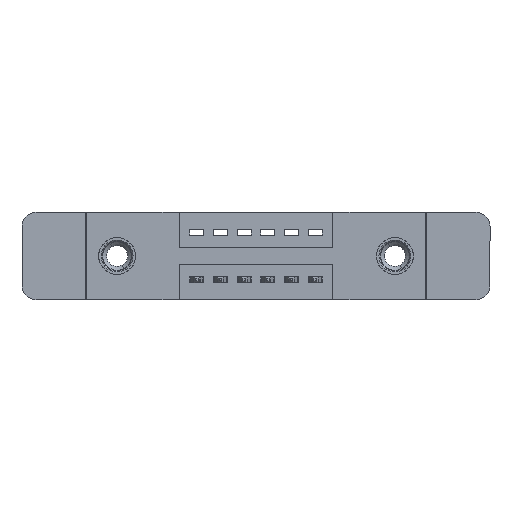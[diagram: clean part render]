
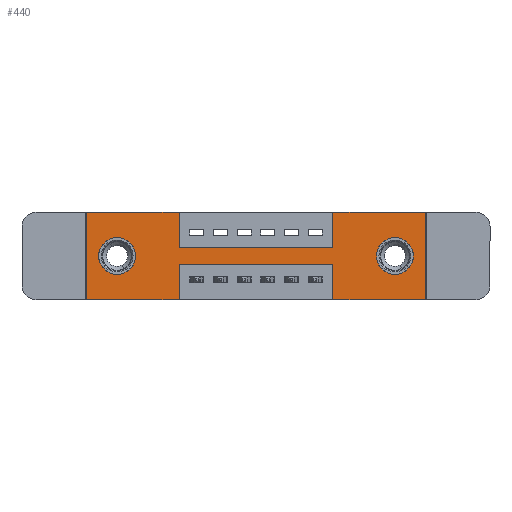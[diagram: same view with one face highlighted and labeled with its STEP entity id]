
A CAD part, front view. The second image highlights one B-rep face of the part: STEP entity #440.
In plain terms, the highlighted planar face has unit normal (0, -1, 0).
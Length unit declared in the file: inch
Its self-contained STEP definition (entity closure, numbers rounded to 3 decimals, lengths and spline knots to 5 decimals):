
#21 = DIRECTION ( 'NONE',  ( 0., 1., 0. ) ) ;
#76 = DIRECTION ( 'NONE',  ( 1., 0., 0. ) ) ;
#92 = CARTESIAN_POINT ( 'NONE',  ( 0.13, 0., -0.107 ) ) ;
#145 = ORIENTED_EDGE ( 'NONE', *, *, #4643, .F. ) ;
#290 = EDGE_CURVE ( 'NONE', #3178, #6219, #2239, .T. ) ;
#355 = CARTESIAN_POINT ( 'NONE',  ( 1.0425, 0., 0. ) ) ;
#369 = EDGE_CURVE ( 'NONE', #3552, #3750, #9083, .T. ) ;
#377 = CARTESIAN_POINT ( 'NONE',  ( 0., 0., -0.37 ) ) ;
#440 = ADVANCED_FACE ( 'NONE', ( #11741, #9780, #4550 ), #5993, .T. ) ;
#637 = CARTESIAN_POINT ( 'NONE',  ( 0.3925, 0., 0. ) ) ;
#699 = ORIENTED_EDGE ( 'NONE', *, *, #4225, .F. ) ;
#749 = DIRECTION ( 'NONE',  ( 0., 0., 1. ) ) ;
#1141 = VERTEX_POINT ( 'NONE', #4146 ) ;
#1316 = CARTESIAN_POINT ( 'NONE',  ( 1.305, 0., -0.185 ) ) ;
#1449 = LINE ( 'NONE', #14171, #9196 ) ;
#1496 = CIRCLE ( 'NONE', #10214, 0.078 ) ;
#1677 = ORIENTED_EDGE ( 'NONE', *, *, #3763, .F. ) ;
#2024 = CARTESIAN_POINT ( 'NONE',  ( 0., 0., -0.37 ) ) ;
#2152 = ORIENTED_EDGE ( 'NONE', *, *, #290, .T. ) ;
#2190 = VECTOR ( 'NONE', #14104, 39.37008 ) ;
#2222 = DIRECTION ( 'NONE',  ( 0., 0., -1. ) ) ;
#2239 = CIRCLE ( 'NONE', #8476, 0.078 ) ;
#2270 = EDGE_CURVE ( 'NONE', #4697, #11535, #8862, .T. ) ;
#2509 = EDGE_CURVE ( 'NONE', #7415, #1141, #1449, .T. ) ;
#2628 = CARTESIAN_POINT ( 'NONE',  ( 0., 0., -0.37 ) ) ;
#2652 = DIRECTION ( 'NONE',  ( 0., -1., 0. ) ) ;
#2662 = LINE ( 'NONE', #14370, #13038 ) ;
#2706 = CARTESIAN_POINT ( 'NONE',  ( 1.435, 0., 0. ) ) ;
#2819 = DIRECTION ( 'NONE',  ( 1., 0., 0. ) ) ;
#2971 = EDGE_CURVE ( 'NONE', #10514, #6165, #10948, .T. ) ;
#2995 = ORIENTED_EDGE ( 'NONE', *, *, #7343, .F. ) ;
#3137 = CARTESIAN_POINT ( 'NONE',  ( 0., 0., 0. ) ) ;
#3178 = VERTEX_POINT ( 'NONE', #6705 ) ;
#3215 = AXIS2_PLACEMENT_3D ( 'NONE', #10278, #21, #9104 ) ;
#3552 = VERTEX_POINT ( 'NONE', #6985 ) ;
#3697 = ORIENTED_EDGE ( 'NONE', *, *, #13777, .F. ) ;
#3750 = VERTEX_POINT ( 'NONE', #9920 ) ;
#3763 = EDGE_CURVE ( 'NONE', #13545, #6543, #2662, .T. ) ;
#3851 = ORIENTED_EDGE ( 'NONE', *, *, #2509, .F. ) ;
#4062 = EDGE_CURVE ( 'NONE', #4641, #10970, #13435, .T. ) ;
#4107 = ORIENTED_EDGE ( 'NONE', *, *, #4062, .F. ) ;
#4146 = CARTESIAN_POINT ( 'NONE',  ( 1.0425, 0., -0.15 ) ) ;
#4225 = EDGE_CURVE ( 'NONE', #6165, #13545, #10480, .T. ) ;
#4286 = VERTEX_POINT ( 'NONE', #5364 ) ;
#4495 = LINE ( 'NONE', #637, #2190 ) ;
#4533 = DIRECTION ( 'NONE',  ( -1., 0., 0. ) ) ;
#4550 = FACE_OUTER_BOUND ( 'NONE', #4663, .T. ) ;
#4641 = VERTEX_POINT ( 'NONE', #12144 ) ;
#4643 = EDGE_CURVE ( 'NONE', #5873, #4641, #6979, .T. ) ;
#4663 = EDGE_LOOP ( 'NONE', ( #1677, #699, #14222, #2995, #6156, #12786, #3697, #3851, #7631, #4107, #145, #11640 ) ) ;
#4697 = VERTEX_POINT ( 'NONE', #6882 ) ;
#4764 = CARTESIAN_POINT ( 'NONE',  ( 1.0425, 0., -0.37 ) ) ;
#4794 = AXIS2_PLACEMENT_3D ( 'NONE', #12573, #5707, #6926 ) ;
#4880 = EDGE_CURVE ( 'NONE', #6219, #3178, #1496, .T. ) ;
#4923 = CARTESIAN_POINT ( 'NONE',  ( 0., 0., -0.37 ) ) ;
#5355 = VECTOR ( 'NONE', #12764, 39.37008 ) ;
#5364 = CARTESIAN_POINT ( 'NONE',  ( 1.0425, 0., 0. ) ) ;
#5394 = DIRECTION ( 'NONE',  ( 0., 0., 1. ) ) ;
#5552 = ORIENTED_EDGE ( 'NONE', *, *, #2270, .T. ) ;
#5650 = EDGE_CURVE ( 'NONE', #11535, #4697, #13793, .T. ) ;
#5707 = DIRECTION ( 'NONE',  ( 0., 1., 0. ) ) ;
#5873 = VERTEX_POINT ( 'NONE', #2628 ) ;
#5907 = CARTESIAN_POINT ( 'NONE',  ( 0.3925, 0., -0.37 ) ) ;
#5952 = DIRECTION ( 'NONE',  ( 0., 1., 0. ) ) ;
#5972 = VECTOR ( 'NONE', #13434, 39.37008 ) ;
#5993 = PLANE ( 'NONE',  #11969 ) ;
#6156 = ORIENTED_EDGE ( 'NONE', *, *, #369, .F. ) ;
#6165 = VERTEX_POINT ( 'NONE', #11853 ) ;
#6219 = VERTEX_POINT ( 'NONE', #8890 ) ;
#6543 = VERTEX_POINT ( 'NONE', #5907 ) ;
#6705 = CARTESIAN_POINT ( 'NONE',  ( 1.305, 0., -0.263 ) ) ;
#6771 = CARTESIAN_POINT ( 'NONE',  ( 0., 0., 0. ) ) ;
#6840 = LINE ( 'NONE', #2024, #5972 ) ;
#6882 = CARTESIAN_POINT ( 'NONE',  ( 0.13, 0., -0.263 ) ) ;
#6926 = DIRECTION ( 'NONE',  ( 0., 0., 1. ) ) ;
#6979 = LINE ( 'NONE', #3137, #13303 ) ;
#6985 = CARTESIAN_POINT ( 'NONE',  ( 1.435, 0., 0. ) ) ;
#7114 = EDGE_LOOP ( 'NONE', ( #10058, #5552 ) ) ;
#7339 = DIRECTION ( 'NONE',  ( 0., 0., -1. ) ) ;
#7343 = EDGE_CURVE ( 'NONE', #3750, #10514, #7796, .T. ) ;
#7346 = DIRECTION ( 'NONE',  ( 0., 1., 0. ) ) ;
#7415 = VERTEX_POINT ( 'NONE', #9679 ) ;
#7631 = ORIENTED_EDGE ( 'NONE', *, *, #14507, .F. ) ;
#7754 = CARTESIAN_POINT ( 'NONE',  ( 0.3925, 0., -0.22 ) ) ;
#7785 = CARTESIAN_POINT ( 'NONE',  ( 0.3925, 0., 0. ) ) ;
#7796 = LINE ( 'NONE', #4923, #5355 ) ;
#7858 = CARTESIAN_POINT ( 'NONE',  ( 1.0425, 0., -0.37 ) ) ;
#7972 = VECTOR ( 'NONE', #11440, 39.37008 ) ;
#8386 = VECTOR ( 'NONE', #10014, 39.37008 ) ;
#8476 = AXIS2_PLACEMENT_3D ( 'NONE', #1316, #5952, #9175 ) ;
#8862 = CIRCLE ( 'NONE', #3215, 0.078 ) ;
#8890 = CARTESIAN_POINT ( 'NONE',  ( 1.305, 0., -0.107 ) ) ;
#9083 = LINE ( 'NONE', #2706, #14013 ) ;
#9104 = DIRECTION ( 'NONE',  ( 0., 0., 1. ) ) ;
#9175 = DIRECTION ( 'NONE',  ( 0., 0., -1. ) ) ;
#9196 = VECTOR ( 'NONE', #2819, 39.37008 ) ;
#9245 = EDGE_CURVE ( 'NONE', #6543, #5873, #6840, .T. ) ;
#9610 = CARTESIAN_POINT ( 'NONE',  ( 1.305, 0., -0.185 ) ) ;
#9679 = CARTESIAN_POINT ( 'NONE',  ( 0.3925, 0., -0.15 ) ) ;
#9780 = FACE_BOUND ( 'NONE', #7114, .T. ) ;
#9920 = CARTESIAN_POINT ( 'NONE',  ( 1.435, 0., -0.37 ) ) ;
#9985 = ORIENTED_EDGE ( 'NONE', *, *, #4880, .T. ) ;
#10014 = DIRECTION ( 'NONE',  ( 1., 0., 0. ) ) ;
#10058 = ORIENTED_EDGE ( 'NONE', *, *, #5650, .T. ) ;
#10066 = VECTOR ( 'NONE', #76, 39.37008 ) ;
#10081 = LINE ( 'NONE', #355, #11332 ) ;
#10214 = AXIS2_PLACEMENT_3D ( 'NONE', #9610, #7346, #14149 ) ;
#10278 = CARTESIAN_POINT ( 'NONE',  ( 0.13, 0., -0.185 ) ) ;
#10414 = EDGE_LOOP ( 'NONE', ( #9985, #2152 ) ) ;
#10480 = LINE ( 'NONE', #14549, #14546 ) ;
#10503 = DIRECTION ( 'NONE',  ( 0., 0., -1. ) ) ;
#10514 = VERTEX_POINT ( 'NONE', #7858 ) ;
#10948 = LINE ( 'NONE', #4764, #7972 ) ;
#10970 = VERTEX_POINT ( 'NONE', #7785 ) ;
#11332 = VECTOR ( 'NONE', #749, 39.37008 ) ;
#11440 = DIRECTION ( 'NONE',  ( 0., 0., 1. ) ) ;
#11535 = VERTEX_POINT ( 'NONE', #92 ) ;
#11640 = ORIENTED_EDGE ( 'NONE', *, *, #9245, .F. ) ;
#11741 = FACE_BOUND ( 'NONE', #10414, .T. ) ;
#11853 = CARTESIAN_POINT ( 'NONE',  ( 1.0425, 0., -0.22 ) ) ;
#11969 = AXIS2_PLACEMENT_3D ( 'NONE', #377, #2652, #10503 ) ;
#12144 = CARTESIAN_POINT ( 'NONE',  ( 0., 0., 0. ) ) ;
#12196 = EDGE_CURVE ( 'NONE', #4286, #3552, #14001, .T. ) ;
#12573 = CARTESIAN_POINT ( 'NONE',  ( 0.13, 0., -0.185 ) ) ;
#12764 = DIRECTION ( 'NONE',  ( -1., 0., 0. ) ) ;
#12786 = ORIENTED_EDGE ( 'NONE', *, *, #12196, .F. ) ;
#13038 = VECTOR ( 'NONE', #2222, 39.37008 ) ;
#13303 = VECTOR ( 'NONE', #5394, 39.37008 ) ;
#13434 = DIRECTION ( 'NONE',  ( -1., 0., 0. ) ) ;
#13435 = LINE ( 'NONE', #6771, #10066 ) ;
#13545 = VERTEX_POINT ( 'NONE', #7754 ) ;
#13777 = EDGE_CURVE ( 'NONE', #1141, #4286, #10081, .T. ) ;
#13793 = CIRCLE ( 'NONE', #4794, 0.078 ) ;
#14001 = LINE ( 'NONE', #14524, #8386 ) ;
#14013 = VECTOR ( 'NONE', #7339, 39.37008 ) ;
#14104 = DIRECTION ( 'NONE',  ( 0., 0., -1. ) ) ;
#14149 = DIRECTION ( 'NONE',  ( 0., 0., -1. ) ) ;
#14171 = CARTESIAN_POINT ( 'NONE',  ( 0.3925, 0., -0.15 ) ) ;
#14222 = ORIENTED_EDGE ( 'NONE', *, *, #2971, .F. ) ;
#14370 = CARTESIAN_POINT ( 'NONE',  ( 0.3925, 0., -0.37 ) ) ;
#14507 = EDGE_CURVE ( 'NONE', #10970, #7415, #4495, .T. ) ;
#14524 = CARTESIAN_POINT ( 'NONE',  ( 0., 0., 0. ) ) ;
#14546 = VECTOR ( 'NONE', #4533, 39.37008 ) ;
#14549 = CARTESIAN_POINT ( 'NONE',  ( 0.3925, 0., -0.22 ) ) ;
